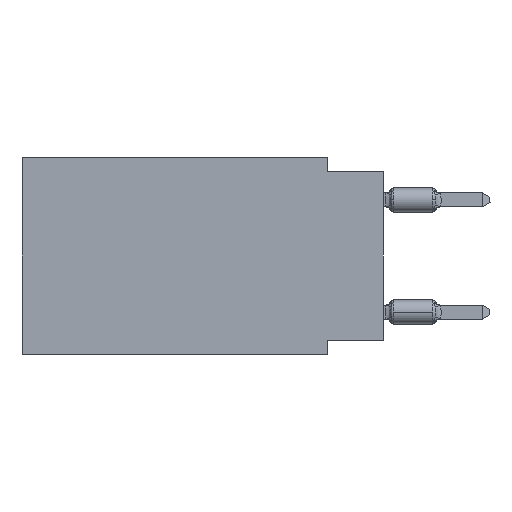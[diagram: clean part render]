
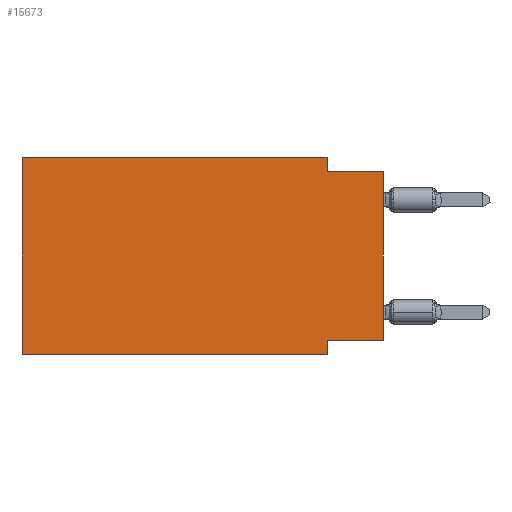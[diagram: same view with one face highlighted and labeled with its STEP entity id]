
A CAD part, left-side view. The second image highlights one B-rep face of the part: STEP entity #15673.
In plain terms, the highlighted planar face has unit normal (-1, 0, 0).
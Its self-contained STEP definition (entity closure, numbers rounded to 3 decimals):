
#238 = CARTESIAN_POINT ( 'NONE',  ( 0., 16.383, -8.89 ) ) ;
#1616 = CARTESIAN_POINT ( 'NONE',  ( 0., 2.54, 0. ) ) ;
#2153 = ORIENTED_EDGE ( 'NONE', *, *, #32714, .F. ) ;
#2365 = ORIENTED_EDGE ( 'NONE', *, *, #48127, .T. ) ;
#3328 = VERTEX_POINT ( 'NONE', #52404 ) ;
#3914 = EDGE_CURVE ( 'NONE', #26760, #29152, #10232, .T. ) ;
#4201 = DIRECTION ( 'NONE',  ( 0., 0., -1. ) ) ;
#6070 = CARTESIAN_POINT ( 'NONE',  ( 0., 0., -8.255 ) ) ;
#7927 = CARTESIAN_POINT ( 'NONE',  ( 0., 0., -0.635 ) ) ;
#9857 = AXIS2_PLACEMENT_3D ( 'NONE', #35733, #53770, #40084 ) ;
#10215 = DIRECTION ( 'NONE',  ( 0., 1., 0. ) ) ;
#10232 = LINE ( 'NONE', #58888, #18854 ) ;
#11623 = VERTEX_POINT ( 'NONE', #38492 ) ;
#12815 = VECTOR ( 'NONE', #13432, 1000. ) ;
#13158 = ORIENTED_EDGE ( 'NONE', *, *, #50042, .F. ) ;
#13253 = EDGE_CURVE ( 'NONE', #11623, #29152, #57353, .T. ) ;
#13432 = DIRECTION ( 'NONE',  ( 0., 0., 1. ) ) ;
#14853 = DIRECTION ( 'NONE',  ( 0., -1., 0. ) ) ;
#15673 = ADVANCED_FACE ( 'NONE', ( #16220 ), #58112, .F. ) ;
#16193 = DIRECTION ( 'NONE',  ( 0., 0., -1. ) ) ;
#16220 = FACE_OUTER_BOUND ( 'NONE', #58548, .T. ) ;
#16388 = EDGE_CURVE ( 'NONE', #26760, #54841, #32528, .T. ) ;
#18854 = VECTOR ( 'NONE', #20750, 1000. ) ;
#20750 = DIRECTION ( 'NONE',  ( 0., 0., 1. ) ) ;
#21230 = ORIENTED_EDGE ( 'NONE', *, *, #16388, .F. ) ;
#21682 = CARTESIAN_POINT ( 'NONE',  ( 0., 2.54, -8.89 ) ) ;
#22209 = VERTEX_POINT ( 'NONE', #21682 ) ;
#22340 = VECTOR ( 'NONE', #29115, 1000. ) ;
#24835 = CARTESIAN_POINT ( 'NONE',  ( 0., 2.54, -8.255 ) ) ;
#26760 = VERTEX_POINT ( 'NONE', #6070 ) ;
#26827 = VECTOR ( 'NONE', #4201, 1000. ) ;
#27002 = ORIENTED_EDGE ( 'NONE', *, *, #3914, .T. ) ;
#27040 = ORIENTED_EDGE ( 'NONE', *, *, #13253, .F. ) ;
#27722 = LINE ( 'NONE', #48424, #28318 ) ;
#28318 = VECTOR ( 'NONE', #46661, 1000. ) ;
#28474 = LINE ( 'NONE', #47723, #22340 ) ;
#28495 = CARTESIAN_POINT ( 'NONE',  ( 0., 0., -0.635 ) ) ;
#29115 = DIRECTION ( 'NONE',  ( 0., -1., 0. ) ) ;
#29152 = VERTEX_POINT ( 'NONE', #7927 ) ;
#30310 = EDGE_CURVE ( 'NONE', #56534, #11623, #44717, .T. ) ;
#31723 = CARTESIAN_POINT ( 'NONE',  ( 0., 16.383, 0. ) ) ;
#32040 = LINE ( 'NONE', #31723, #12815 ) ;
#32528 = LINE ( 'NONE', #56119, #60007 ) ;
#32714 = EDGE_CURVE ( 'NONE', #34485, #3328, #32040, .T. ) ;
#34485 = VERTEX_POINT ( 'NONE', #238 ) ;
#35623 = CARTESIAN_POINT ( 'NONE',  ( 0., 2.54, -8.89 ) ) ;
#35733 = CARTESIAN_POINT ( 'NONE',  ( 0., 16.383, 0. ) ) ;
#35983 = VECTOR ( 'NONE', #16193, 1000. ) ;
#38492 = CARTESIAN_POINT ( 'NONE',  ( 0., 2.54, -0.635 ) ) ;
#40084 = DIRECTION ( 'NONE',  ( 0., 0., -1. ) ) ;
#40248 = CARTESIAN_POINT ( 'NONE',  ( 0., 2.54, 0. ) ) ;
#44195 = ORIENTED_EDGE ( 'NONE', *, *, #57675, .F. ) ;
#44717 = LINE ( 'NONE', #1616, #35983 ) ;
#46606 = VECTOR ( 'NONE', #14853, 1000. ) ;
#46661 = DIRECTION ( 'NONE',  ( 0., -1., 0. ) ) ;
#47723 = CARTESIAN_POINT ( 'NONE',  ( 0., 16.383, 0. ) ) ;
#48127 = EDGE_CURVE ( 'NONE', #34485, #22209, #27722, .T. ) ;
#48424 = CARTESIAN_POINT ( 'NONE',  ( 0., 16.383, -8.89 ) ) ;
#50042 = EDGE_CURVE ( 'NONE', #3328, #56534, #28474, .T. ) ;
#52404 = CARTESIAN_POINT ( 'NONE',  ( 0., 16.383, 0. ) ) ;
#53770 = DIRECTION ( 'NONE',  ( 1., 0., 0. ) ) ;
#54841 = VERTEX_POINT ( 'NONE', #24835 ) ;
#55525 = ORIENTED_EDGE ( 'NONE', *, *, #30310, .F. ) ;
#56013 = LINE ( 'NONE', #35623, #26827 ) ;
#56119 = CARTESIAN_POINT ( 'NONE',  ( 0., 0., -8.255 ) ) ;
#56534 = VERTEX_POINT ( 'NONE', #40248 ) ;
#57353 = LINE ( 'NONE', #28495, #46606 ) ;
#57675 = EDGE_CURVE ( 'NONE', #54841, #22209, #56013, .T. ) ;
#58112 = PLANE ( 'NONE',  #9857 ) ;
#58548 = EDGE_LOOP ( 'NONE', ( #27002, #27040, #55525, #13158, #2153, #2365, #44195, #21230 ) ) ;
#58888 = CARTESIAN_POINT ( 'NONE',  ( 0., 0., 0. ) ) ;
#60007 = VECTOR ( 'NONE', #10215, 1000. ) ;
